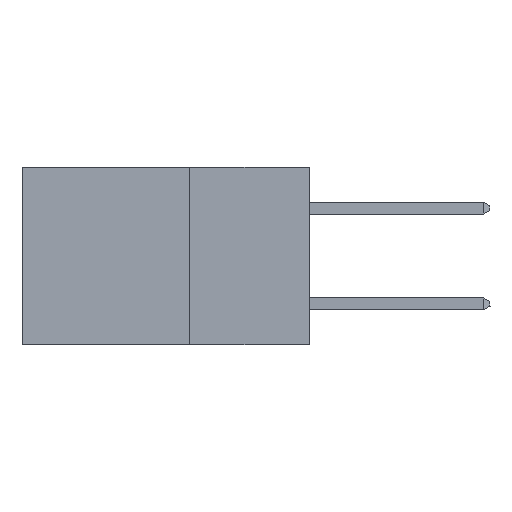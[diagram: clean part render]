
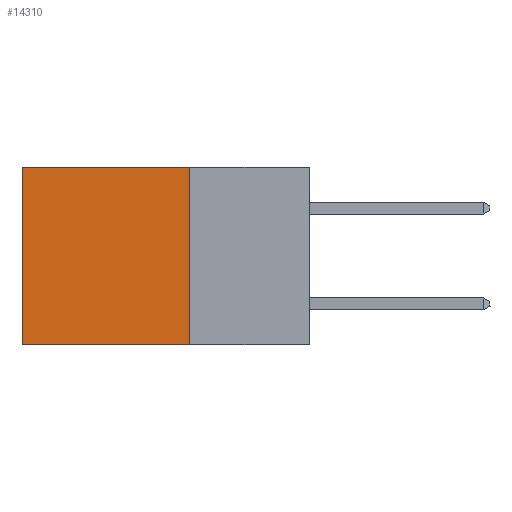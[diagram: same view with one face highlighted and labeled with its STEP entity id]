
A CAD part, left-side view. The second image highlights one B-rep face of the part: STEP entity #14310.
In plain terms, the highlighted planar face has unit normal (-1, 0, 0).
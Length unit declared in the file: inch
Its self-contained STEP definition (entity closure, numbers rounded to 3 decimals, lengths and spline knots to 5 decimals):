
#224 = CARTESIAN_POINT ( 'NONE',  ( 0.2875, 0.25, -0.37 ) ) ;
#267 = ORIENTED_EDGE ( 'NONE', *, *, #7519, .F. ) ;
#1367 = CARTESIAN_POINT ( 'NONE',  ( 0.2875, 0.25, 0. ) ) ;
#1535 = DIRECTION ( 'NONE',  ( 0., 0., -1. ) ) ;
#3047 = CARTESIAN_POINT ( 'NONE',  ( 0.2875, 0.6, -0.37 ) ) ;
#3848 = VERTEX_POINT ( 'NONE', #13206 ) ;
#4509 = EDGE_LOOP ( 'NONE', ( #4604, #19756, #267, #13973 ) ) ;
#4604 = ORIENTED_EDGE ( 'NONE', *, *, #13247, .T. ) ;
#5347 = LINE ( 'NONE', #21086, #15125 ) ;
#5784 = PLANE ( 'NONE',  #21576 ) ;
#5959 = CARTESIAN_POINT ( 'NONE',  ( 0.2875, 0.25, 0. ) ) ;
#6122 = EDGE_CURVE ( 'NONE', #8369, #8310, #10238, .T. ) ;
#7370 = DIRECTION ( 'NONE',  ( 0., 1., 0. ) ) ;
#7519 = EDGE_CURVE ( 'NONE', #9307, #8369, #22685, .T. ) ;
#8310 = VERTEX_POINT ( 'NONE', #3047 ) ;
#8369 = VERTEX_POINT ( 'NONE', #224 ) ;
#8646 = LINE ( 'NONE', #14895, #10920 ) ;
#9307 = VERTEX_POINT ( 'NONE', #1367 ) ;
#9325 = CARTESIAN_POINT ( 'NONE',  ( 0.2875, 0.25, -0.37 ) ) ;
#9338 = DIRECTION ( 'NONE',  ( 0., 0., -1. ) ) ;
#9944 = VECTOR ( 'NONE', #7370, 39.37008 ) ;
#10238 = LINE ( 'NONE', #9325, #9944 ) ;
#10920 = VECTOR ( 'NONE', #25436, 39.37008 ) ;
#10944 = DIRECTION ( 'NONE',  ( 0., 0., -1. ) ) ;
#11113 = CARTESIAN_POINT ( 'NONE',  ( 0.2875, 0.25, 0. ) ) ;
#12104 = EDGE_CURVE ( 'NONE', #9307, #3848, #8646, .T. ) ;
#13206 = CARTESIAN_POINT ( 'NONE',  ( 0.2875, 0.6, 0. ) ) ;
#13247 = EDGE_CURVE ( 'NONE', #3848, #8310, #5347, .T. ) ;
#13973 = ORIENTED_EDGE ( 'NONE', *, *, #12104, .T. ) ;
#14249 = DIRECTION ( 'NONE',  ( 1., 0., 0. ) ) ;
#14310 = ADVANCED_FACE ( 'NONE', ( #23595 ), #5784, .F. ) ;
#14895 = CARTESIAN_POINT ( 'NONE',  ( 0.2875, 0.25, 0. ) ) ;
#15125 = VECTOR ( 'NONE', #9338, 39.37008 ) ;
#19756 = ORIENTED_EDGE ( 'NONE', *, *, #6122, .F. ) ;
#20733 = VECTOR ( 'NONE', #10944, 39.37008 ) ;
#21086 = CARTESIAN_POINT ( 'NONE',  ( 0.2875, 0.6, 0. ) ) ;
#21576 = AXIS2_PLACEMENT_3D ( 'NONE', #5959, #14249, #1535 ) ;
#22685 = LINE ( 'NONE', #11113, #20733 ) ;
#23595 = FACE_OUTER_BOUND ( 'NONE', #4509, .T. ) ;
#25436 = DIRECTION ( 'NONE',  ( 0., 1., 0. ) ) ;
